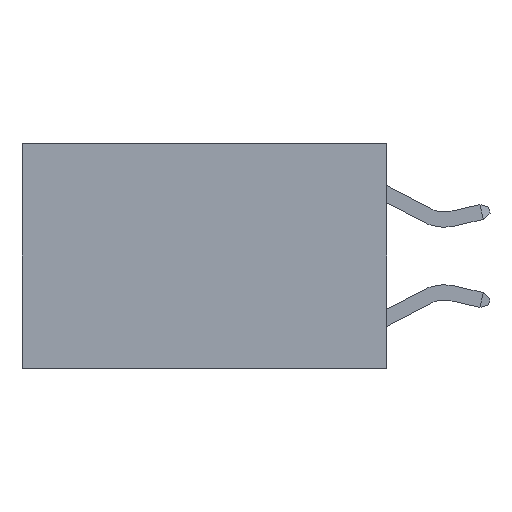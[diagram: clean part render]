
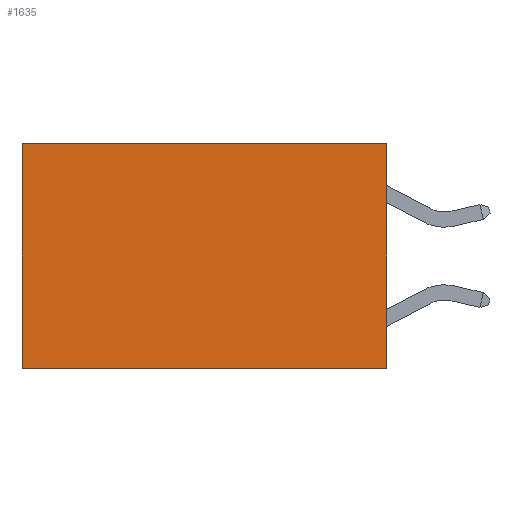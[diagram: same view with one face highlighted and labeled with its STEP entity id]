
A CAD part, left-side view. The second image highlights one B-rep face of the part: STEP entity #1635.
In plain terms, the highlighted planar face has unit normal (-1, 0, 0).
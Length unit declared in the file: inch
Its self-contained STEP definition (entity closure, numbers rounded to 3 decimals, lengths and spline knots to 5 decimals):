
#11 = ORIENTED_EDGE ( 'NONE', *, *, #6722, .T. ) ;
#295 = DIRECTION ( 'NONE',  ( 0., 0., -1. ) ) ;
#505 = VERTEX_POINT ( 'NONE', #1664 ) ;
#640 = ORIENTED_EDGE ( 'NONE', *, *, #7021, .F. ) ;
#913 = VERTEX_POINT ( 'NONE', #2606 ) ;
#994 = FACE_OUTER_BOUND ( 'NONE', #5456, .T. ) ;
#1044 = ORIENTED_EDGE ( 'NONE', *, *, #6406, .F. ) ;
#1258 = CARTESIAN_POINT ( 'NONE',  ( 0.2625, 0., 0. ) ) ;
#1543 = LINE ( 'NONE', #6107, #7640 ) ;
#1635 = ADVANCED_FACE ( 'NONE', ( #994 ), #7113, .F. ) ;
#1664 = CARTESIAN_POINT ( 'NONE',  ( 0.2625, 0.6, 0. ) ) ;
#1755 = LINE ( 'NONE', #8148, #8613 ) ;
#1884 = VERTEX_POINT ( 'NONE', #7604 ) ;
#1909 = CARTESIAN_POINT ( 'NONE',  ( 0.2625, 0., 0. ) ) ;
#2606 = CARTESIAN_POINT ( 'NONE',  ( 0.2625, 0.6, -0.37 ) ) ;
#2782 = DIRECTION ( 'NONE',  ( 0., 0., -1. ) ) ;
#3166 = AXIS2_PLACEMENT_3D ( 'NONE', #1909, #6539, #295 ) ;
#3533 = ORIENTED_EDGE ( 'NONE', *, *, #7272, .T. ) ;
#3663 = VECTOR ( 'NONE', #4431, 39.37008 ) ;
#4051 = DIRECTION ( 'NONE',  ( 0., 0., -1. ) ) ;
#4142 = VERTEX_POINT ( 'NONE', #8459 ) ;
#4431 = DIRECTION ( 'NONE',  ( 0., 1., 0. ) ) ;
#5456 = EDGE_LOOP ( 'NONE', ( #3533, #640, #1044, #11 ) ) ;
#6057 = LINE ( 'NONE', #6543, #3663 ) ;
#6107 = CARTESIAN_POINT ( 'NONE',  ( 0.2625, 0.6, 0. ) ) ;
#6175 = VECTOR ( 'NONE', #4051, 39.37008 ) ;
#6297 = LINE ( 'NONE', #1258, #6175 ) ;
#6406 = EDGE_CURVE ( 'NONE', #1884, #4142, #6297, .T. ) ;
#6539 = DIRECTION ( 'NONE',  ( 1., 0., 0. ) ) ;
#6543 = CARTESIAN_POINT ( 'NONE',  ( 0.2625, 0., -0.37 ) ) ;
#6722 = EDGE_CURVE ( 'NONE', #1884, #505, #1755, .T. ) ;
#7021 = EDGE_CURVE ( 'NONE', #4142, #913, #6057, .T. ) ;
#7113 = PLANE ( 'NONE',  #3166 ) ;
#7272 = EDGE_CURVE ( 'NONE', #505, #913, #1543, .T. ) ;
#7466 = DIRECTION ( 'NONE',  ( 0., 1., 0. ) ) ;
#7604 = CARTESIAN_POINT ( 'NONE',  ( 0.2625, 0., 0. ) ) ;
#7640 = VECTOR ( 'NONE', #2782, 39.37008 ) ;
#8148 = CARTESIAN_POINT ( 'NONE',  ( 0.2625, 0., 0. ) ) ;
#8459 = CARTESIAN_POINT ( 'NONE',  ( 0.2625, 0., -0.37 ) ) ;
#8613 = VECTOR ( 'NONE', #7466, 39.37008 ) ;
